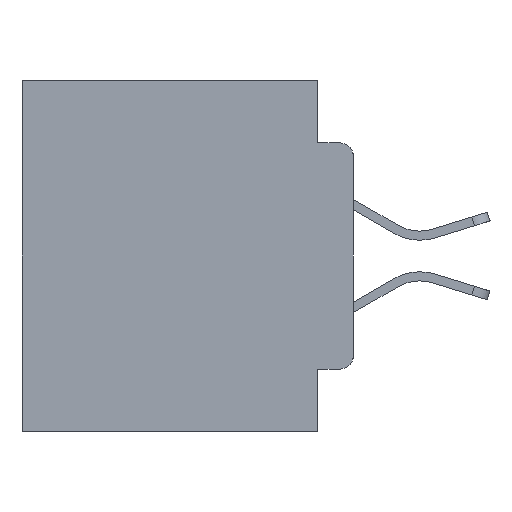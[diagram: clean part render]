
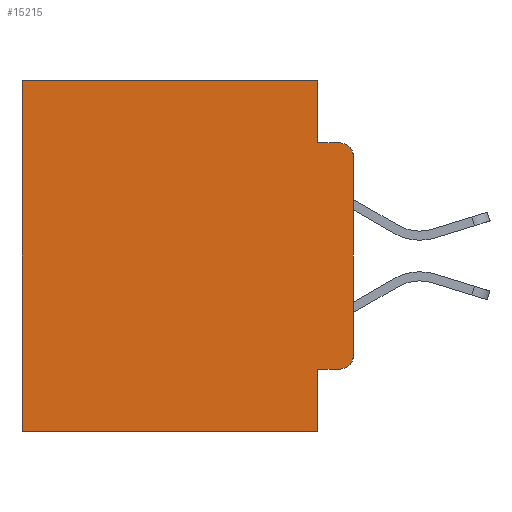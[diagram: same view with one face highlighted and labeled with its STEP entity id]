
A CAD part, left-side view. The second image highlights one B-rep face of the part: STEP entity #15215.
In plain terms, the highlighted planar face has unit normal (-1, 0, 0).
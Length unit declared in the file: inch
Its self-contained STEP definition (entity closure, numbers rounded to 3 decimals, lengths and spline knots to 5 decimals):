
#163 = AXIS2_PLACEMENT_3D ( 'NONE', #24645, #12356, #26640 ) ;
#191 = EDGE_CURVE ( 'NONE', #6084, #10416, #2886, .T. ) ;
#795 = VERTEX_POINT ( 'NONE', #4124 ) ;
#1162 = VERTEX_POINT ( 'NONE', #24370 ) ;
#1439 = VERTEX_POINT ( 'NONE', #14834 ) ;
#1530 = DIRECTION ( 'NONE',  ( 0., 0., -1. ) ) ;
#1767 = CARTESIAN_POINT ( 'NONE',  ( 0.298, 0.051, 0. ) ) ;
#2128 = DIRECTION ( 'NONE',  ( 0., 0., -1. ) ) ;
#2229 = AXIS2_PLACEMENT_3D ( 'NONE', #26304, #14127, #1530 ) ;
#2650 = ORIENTED_EDGE ( 'NONE', *, *, #191, .F. ) ;
#2886 = LINE ( 'NONE', #26331, #24291 ) ;
#2907 = LINE ( 'NONE', #22416, #7828 ) ;
#4124 = CARTESIAN_POINT ( 'NONE',  ( 0.298, 0.02, -0.0885 ) ) ;
#5001 = PLANE ( 'NONE',  #18677 ) ;
#5111 = LINE ( 'NONE', #20331, #15596 ) ;
#6084 = VERTEX_POINT ( 'NONE', #22990 ) ;
#6444 = DIRECTION ( 'NONE',  ( 0., 0., -1. ) ) ;
#6549 = LINE ( 'NONE', #12374, #7185 ) ;
#6553 = EDGE_CURVE ( 'NONE', #11184, #795, #2907, .T. ) ;
#6676 = VECTOR ( 'NONE', #13047, 39.37008 ) ;
#6934 = ORIENTED_EDGE ( 'NONE', *, *, #6553, .F. ) ;
#7183 = DIRECTION ( 'NONE',  ( 0., 0., -1. ) ) ;
#7185 = VECTOR ( 'NONE', #14497, 39.37008 ) ;
#7495 = VERTEX_POINT ( 'NONE', #21022 ) ;
#7575 = ORIENTED_EDGE ( 'NONE', *, *, #22506, .T. ) ;
#7828 = VECTOR ( 'NONE', #14271, 39.37008 ) ;
#7982 = LINE ( 'NONE', #10924, #6676 ) ;
#8055 = VERTEX_POINT ( 'NONE', #1767 ) ;
#8158 = EDGE_CURVE ( 'NONE', #8055, #11184, #12550, .T. ) ;
#10416 = VERTEX_POINT ( 'NONE', #21932 ) ;
#10456 = CARTESIAN_POINT ( 'NONE',  ( 0.298, 0.02, -0.4115 ) ) ;
#10924 = CARTESIAN_POINT ( 'NONE',  ( 0.298, 0.473, 0. ) ) ;
#11184 = VERTEX_POINT ( 'NONE', #12353 ) ;
#12353 = CARTESIAN_POINT ( 'NONE',  ( 0.298, 0.051, -0.0885 ) ) ;
#12356 = DIRECTION ( 'NONE',  ( -1., 0., 0. ) ) ;
#12374 = CARTESIAN_POINT ( 'NONE',  ( 0.298, 0.051, -0.4115 ) ) ;
#12550 = LINE ( 'NONE', #14708, #17392 ) ;
#13047 = DIRECTION ( 'NONE',  ( 0., 0., -1. ) ) ;
#13273 = EDGE_LOOP ( 'NONE', ( #17366, #14061, #6934, #18251, #7575, #18589, #24012, #2650, #13749, #22511 ) ) ;
#13287 = LINE ( 'NONE', #19250, #23565 ) ;
#13566 = CARTESIAN_POINT ( 'NONE',  ( 0.298, 0., 0. ) ) ;
#13749 = ORIENTED_EDGE ( 'NONE', *, *, #26065, .T. ) ;
#14061 = ORIENTED_EDGE ( 'NONE', *, *, #19259, .T. ) ;
#14127 = DIRECTION ( 'NONE',  ( -1., 0., 0. ) ) ;
#14133 = DIRECTION ( 'NONE',  ( 0., 1., 0. ) ) ;
#14271 = DIRECTION ( 'NONE',  ( 0., -1., 0. ) ) ;
#14497 = DIRECTION ( 'NONE',  ( 0., -1., 0. ) ) ;
#14708 = CARTESIAN_POINT ( 'NONE',  ( 0.298, 0.051, 0. ) ) ;
#14834 = CARTESIAN_POINT ( 'NONE',  ( 0.298, 0.473, 0. ) ) ;
#15215 = ADVANCED_FACE ( 'NONE', ( #19911 ), #5001, .F. ) ;
#15596 = VECTOR ( 'NONE', #14133, 39.37008 ) ;
#17366 = ORIENTED_EDGE ( 'NONE', *, *, #19022, .F. ) ;
#17392 = VECTOR ( 'NONE', #2128, 39.37008 ) ;
#18251 = ORIENTED_EDGE ( 'NONE', *, *, #8158, .F. ) ;
#18517 = VERTEX_POINT ( 'NONE', #23985 ) ;
#18589 = ORIENTED_EDGE ( 'NONE', *, *, #23924, .T. ) ;
#18677 = AXIS2_PLACEMENT_3D ( 'NONE', #25658, #19661, #7183 ) ;
#18860 = EDGE_CURVE ( 'NONE', #10416, #1162, #13287, .T. ) ;
#19022 = EDGE_CURVE ( 'NONE', #18517, #7495, #20375, .T. ) ;
#19250 = CARTESIAN_POINT ( 'NONE',  ( 0.298, 0., -0.5 ) ) ;
#19259 = EDGE_CURVE ( 'NONE', #18517, #795, #24786, .T. ) ;
#19661 = DIRECTION ( 'NONE',  ( 1., 0., 0. ) ) ;
#19911 = FACE_OUTER_BOUND ( 'NONE', #13273, .T. ) ;
#20331 = CARTESIAN_POINT ( 'NONE',  ( 0.298, 0., 0. ) ) ;
#20375 = LINE ( 'NONE', #13566, #25114 ) ;
#20858 = CIRCLE ( 'NONE', #2229, 0.02 ) ;
#21022 = CARTESIAN_POINT ( 'NONE',  ( 0.298, 0., -0.3915 ) ) ;
#21932 = CARTESIAN_POINT ( 'NONE',  ( 0.298, 0.051, -0.5 ) ) ;
#22416 = CARTESIAN_POINT ( 'NONE',  ( 0.298, 0.051, -0.0885 ) ) ;
#22506 = EDGE_CURVE ( 'NONE', #8055, #1439, #5111, .T. ) ;
#22511 = ORIENTED_EDGE ( 'NONE', *, *, #25935, .T. ) ;
#22643 = VERTEX_POINT ( 'NONE', #10456 ) ;
#22990 = CARTESIAN_POINT ( 'NONE',  ( 0.298, 0.051, -0.4115 ) ) ;
#23352 = DIRECTION ( 'NONE',  ( 0., 1., 0. ) ) ;
#23565 = VECTOR ( 'NONE', #23352, 39.37008 ) ;
#23794 = DIRECTION ( 'NONE',  ( 0., 0., -1. ) ) ;
#23924 = EDGE_CURVE ( 'NONE', #1439, #1162, #7982, .T. ) ;
#23985 = CARTESIAN_POINT ( 'NONE',  ( 0.298, 0., -0.1085 ) ) ;
#24012 = ORIENTED_EDGE ( 'NONE', *, *, #18860, .F. ) ;
#24291 = VECTOR ( 'NONE', #6444, 39.37008 ) ;
#24370 = CARTESIAN_POINT ( 'NONE',  ( 0.298, 0.473, -0.5 ) ) ;
#24645 = CARTESIAN_POINT ( 'NONE',  ( 0.298, 0.02, -0.1085 ) ) ;
#24786 = CIRCLE ( 'NONE', #163, 0.02 ) ;
#25114 = VECTOR ( 'NONE', #23794, 39.37008 ) ;
#25658 = CARTESIAN_POINT ( 'NONE',  ( 0.298, 0., 0. ) ) ;
#25935 = EDGE_CURVE ( 'NONE', #22643, #7495, #20858, .T. ) ;
#26065 = EDGE_CURVE ( 'NONE', #6084, #22643, #6549, .T. ) ;
#26304 = CARTESIAN_POINT ( 'NONE',  ( 0.298, 0.02, -0.3915 ) ) ;
#26331 = CARTESIAN_POINT ( 'NONE',  ( 0.298, 0.051, 0. ) ) ;
#26640 = DIRECTION ( 'NONE',  ( 0., 0., -1. ) ) ;
